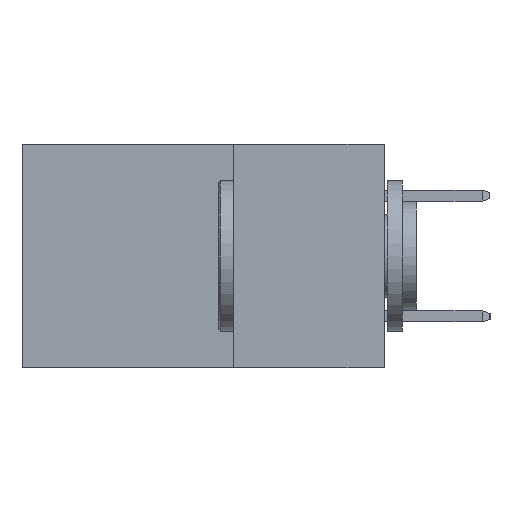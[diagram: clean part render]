
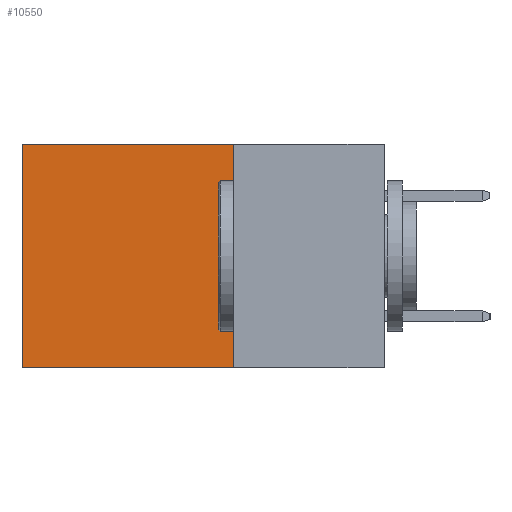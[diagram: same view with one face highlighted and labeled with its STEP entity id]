
A CAD part, left-side view. The second image highlights one B-rep face of the part: STEP entity #10550.
In plain terms, the highlighted planar face has unit normal (-1, 0, 0).
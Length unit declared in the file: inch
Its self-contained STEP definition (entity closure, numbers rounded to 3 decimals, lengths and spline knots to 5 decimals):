
#1176 = ORIENTED_EDGE ( 'NONE', *, *, #2238, .F. ) ;
#2123 = LINE ( 'NONE', #10082, #12329 ) ;
#2238 = EDGE_CURVE ( 'NONE', #9803, #5154, #2123, .T. ) ;
#2518 = CARTESIAN_POINT ( 'NONE',  ( 0.2615, 0.6, 0. ) ) ;
#2722 = CARTESIAN_POINT ( 'NONE',  ( 0.2615, 0.25, -0.37 ) ) ;
#2855 = DIRECTION ( 'NONE',  ( 0., 1., 0. ) ) ;
#2867 = VERTEX_POINT ( 'NONE', #2518 ) ;
#3750 = FACE_OUTER_BOUND ( 'NONE', #3939, .T. ) ;
#3939 = EDGE_LOOP ( 'NONE', ( #7394, #8103, #1176, #4176 ) ) ;
#4176 = ORIENTED_EDGE ( 'NONE', *, *, #10701, .T. ) ;
#4921 = PLANE ( 'NONE',  #6745 ) ;
#5154 = VERTEX_POINT ( 'NONE', #9785 ) ;
#5173 = CARTESIAN_POINT ( 'NONE',  ( 0.2615, 0.25, 0. ) ) ;
#5799 = EDGE_CURVE ( 'NONE', #5154, #10237, #12411, .T. ) ;
#5951 = DIRECTION ( 'NONE',  ( 0., 0., -1. ) ) ;
#6237 = DIRECTION ( 'NONE',  ( 0., 1., 0. ) ) ;
#6639 = CARTESIAN_POINT ( 'NONE',  ( 0.2615, 0.25, 0. ) ) ;
#6745 = AXIS2_PLACEMENT_3D ( 'NONE', #9882, #11811, #5951 ) ;
#7394 = ORIENTED_EDGE ( 'NONE', *, *, #10994, .T. ) ;
#7571 = DIRECTION ( 'NONE',  ( 0., 0., -1. ) ) ;
#8103 = ORIENTED_EDGE ( 'NONE', *, *, #5799, .F. ) ;
#8281 = DIRECTION ( 'NONE',  ( 0., 0., -1. ) ) ;
#9075 = VECTOR ( 'NONE', #7571, 39.37008 ) ;
#9385 = LINE ( 'NONE', #9527, #9075 ) ;
#9527 = CARTESIAN_POINT ( 'NONE',  ( 0.2615, 0.6, -0.37 ) ) ;
#9785 = CARTESIAN_POINT ( 'NONE',  ( 0.2615, 0.25, -0.37 ) ) ;
#9803 = VERTEX_POINT ( 'NONE', #6639 ) ;
#9866 = VECTOR ( 'NONE', #2855, 39.37008 ) ;
#9882 = CARTESIAN_POINT ( 'NONE',  ( 0.2615, 0.25, -0.37 ) ) ;
#10082 = CARTESIAN_POINT ( 'NONE',  ( 0.2615, 0.25, -0.37 ) ) ;
#10164 = LINE ( 'NONE', #5173, #12101 ) ;
#10200 = CARTESIAN_POINT ( 'NONE',  ( 0.2615, 0.6, -0.37 ) ) ;
#10237 = VERTEX_POINT ( 'NONE', #10200 ) ;
#10550 = ADVANCED_FACE ( 'NONE', ( #3750 ), #4921, .F. ) ;
#10701 = EDGE_CURVE ( 'NONE', #9803, #2867, #10164, .T. ) ;
#10994 = EDGE_CURVE ( 'NONE', #2867, #10237, #9385, .T. ) ;
#11811 = DIRECTION ( 'NONE',  ( 1., 0., 0. ) ) ;
#12101 = VECTOR ( 'NONE', #6237, 39.37008 ) ;
#12329 = VECTOR ( 'NONE', #8281, 39.37008 ) ;
#12411 = LINE ( 'NONE', #2722, #9866 ) ;
